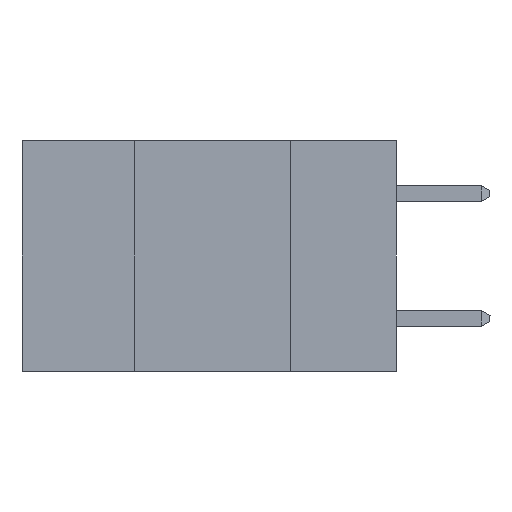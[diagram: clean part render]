
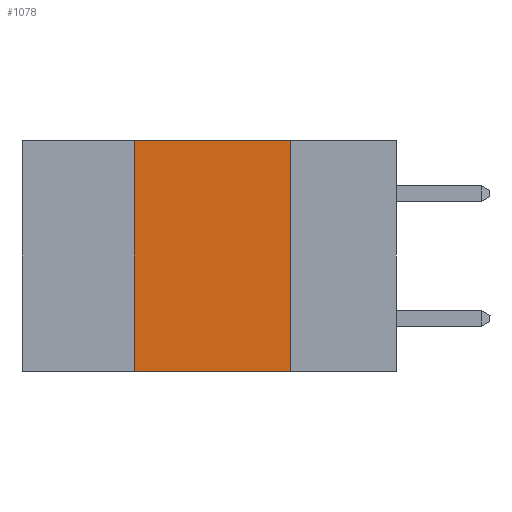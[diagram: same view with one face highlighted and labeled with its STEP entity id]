
A CAD part, left-side view. The second image highlights one B-rep face of the part: STEP entity #1078.
In plain terms, the highlighted planar face has unit normal (-1, 0, 0).
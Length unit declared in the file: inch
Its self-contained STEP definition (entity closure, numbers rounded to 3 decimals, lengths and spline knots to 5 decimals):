
#219 = CARTESIAN_POINT ( 'NONE',  ( 0., 0.17, 0. ) ) ;
#438 = VECTOR ( 'NONE', #5608, 39.37008 ) ;
#620 = CARTESIAN_POINT ( 'NONE',  ( 0., 0.17, -0.37 ) ) ;
#635 = VERTEX_POINT ( 'NONE', #620 ) ;
#909 = VECTOR ( 'NONE', #4421, 39.37008 ) ;
#1025 = DIRECTION ( 'NONE',  ( 1., 0., 0. ) ) ;
#1078 = ADVANCED_FACE ( 'NONE', ( #8620 ), #1351, .F. ) ;
#1229 = VERTEX_POINT ( 'NONE', #3091 ) ;
#1351 = PLANE ( 'NONE',  #7606 ) ;
#1796 = ORIENTED_EDGE ( 'NONE', *, *, #4723, .F. ) ;
#1873 = VECTOR ( 'NONE', #4932, 39.37008 ) ;
#2211 = ORIENTED_EDGE ( 'NONE', *, *, #3329, .F. ) ;
#2219 = ORIENTED_EDGE ( 'NONE', *, *, #3790, .F. ) ;
#2332 = EDGE_CURVE ( 'NONE', #8572, #635, #6618, .T. ) ;
#2564 = LINE ( 'NONE', #5358, #438 ) ;
#2789 = DIRECTION ( 'NONE',  ( 0., 0., -1. ) ) ;
#2862 = VERTEX_POINT ( 'NONE', #219 ) ;
#3091 = CARTESIAN_POINT ( 'NONE',  ( 0., 0.42, 0. ) ) ;
#3194 = DIRECTION ( 'NONE',  ( 0., -1., 0. ) ) ;
#3195 = CARTESIAN_POINT ( 'NONE',  ( 0., 0.6, 0. ) ) ;
#3329 = EDGE_CURVE ( 'NONE', #8572, #1229, #2564, .T. ) ;
#3790 = EDGE_CURVE ( 'NONE', #1229, #2862, #5853, .T. ) ;
#3800 = VECTOR ( 'NONE', #3194, 39.37008 ) ;
#4384 = CARTESIAN_POINT ( 'NONE',  ( 0., 0.6, -0.37 ) ) ;
#4421 = DIRECTION ( 'NONE',  ( 0., -1., 0. ) ) ;
#4723 = EDGE_CURVE ( 'NONE', #2862, #635, #7217, .T. ) ;
#4932 = DIRECTION ( 'NONE',  ( 0., 0., -1. ) ) ;
#4977 = CARTESIAN_POINT ( 'NONE',  ( 0., 0.17, -0.37 ) ) ;
#5358 = CARTESIAN_POINT ( 'NONE',  ( 0., 0.42, -0.37 ) ) ;
#5608 = DIRECTION ( 'NONE',  ( 0., 0., 1. ) ) ;
#5853 = LINE ( 'NONE', #3195, #3800 ) ;
#6618 = LINE ( 'NONE', #4384, #909 ) ;
#6981 = CARTESIAN_POINT ( 'NONE',  ( 0., 0.42, -0.37 ) ) ;
#7217 = LINE ( 'NONE', #4977, #1873 ) ;
#7606 = AXIS2_PLACEMENT_3D ( 'NONE', #7972, #1025, #2789 ) ;
#7972 = CARTESIAN_POINT ( 'NONE',  ( 0., 0.6, 0. ) ) ;
#8063 = EDGE_LOOP ( 'NONE', ( #1796, #2219, #2211, #8345 ) ) ;
#8345 = ORIENTED_EDGE ( 'NONE', *, *, #2332, .T. ) ;
#8572 = VERTEX_POINT ( 'NONE', #6981 ) ;
#8620 = FACE_OUTER_BOUND ( 'NONE', #8063, .T. ) ;
